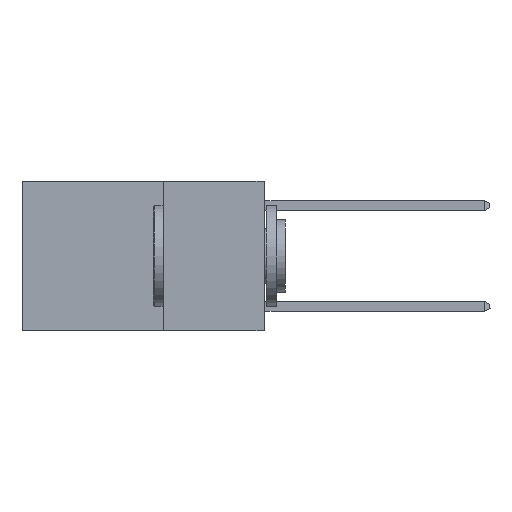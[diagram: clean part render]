
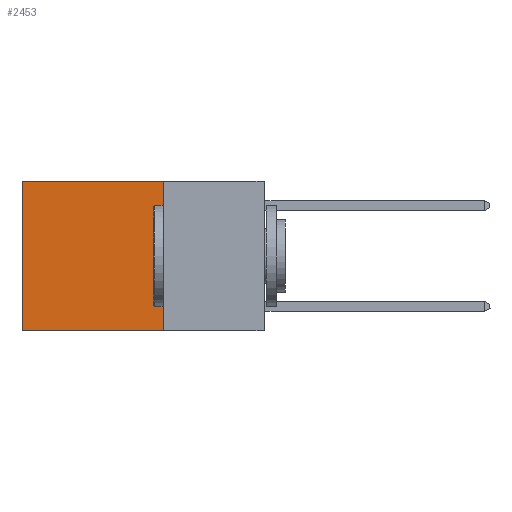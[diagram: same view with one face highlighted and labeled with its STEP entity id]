
A CAD part, left-side view. The second image highlights one B-rep face of the part: STEP entity #2453.
In plain terms, the highlighted planar face has unit normal (-1, 0, 0).
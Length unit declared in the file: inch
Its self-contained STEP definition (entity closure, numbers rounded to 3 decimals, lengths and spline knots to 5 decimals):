
#381 = DIRECTION ( 'NONE',  ( 1., 0., 0. ) ) ;
#887 = ORIENTED_EDGE ( 'NONE', *, *, #4737, .F. ) ;
#996 = LINE ( 'NONE', #11711, #10365 ) ;
#1130 = LINE ( 'NONE', #4098, #22455 ) ;
#1272 = CARTESIAN_POINT ( 'NONE',  ( 0.2625, 0.6, -0.37 ) ) ;
#1273 = CARTESIAN_POINT ( 'NONE',  ( 0.2625, 0.25, -0.37 ) ) ;
#1328 = CARTESIAN_POINT ( 'NONE',  ( 0.2625, 0.25, 0. ) ) ;
#2014 = FACE_OUTER_BOUND ( 'NONE', #2048, .T. ) ;
#2048 = EDGE_LOOP ( 'NONE', ( #14635, #13469, #887, #3648 ) ) ;
#2453 = ADVANCED_FACE ( 'NONE', ( #2014 ), #11058, .F. ) ;
#3527 = LINE ( 'NONE', #1328, #14250 ) ;
#3648 = ORIENTED_EDGE ( 'NONE', *, *, #15395, .T. ) ;
#4098 = CARTESIAN_POINT ( 'NONE',  ( 0.2625, 0.6, 0. ) ) ;
#4127 = VERTEX_POINT ( 'NONE', #8095 ) ;
#4737 = EDGE_CURVE ( 'NONE', #4127, #12629, #3527, .T. ) ;
#8095 = CARTESIAN_POINT ( 'NONE',  ( 0.2625, 0.25, 0. ) ) ;
#8576 = CARTESIAN_POINT ( 'NONE',  ( 0.2625, 0.6, 0. ) ) ;
#9661 = DIRECTION ( 'NONE',  ( 0., 1., 0. ) ) ;
#9745 = VERTEX_POINT ( 'NONE', #1272 ) ;
#9850 = DIRECTION ( 'NONE',  ( 0., 0., -1. ) ) ;
#10365 = VECTOR ( 'NONE', #9661, 39.37008 ) ;
#11058 = PLANE ( 'NONE',  #26579 ) ;
#11082 = DIRECTION ( 'NONE',  ( 0., 1., 0. ) ) ;
#11711 = CARTESIAN_POINT ( 'NONE',  ( 0.2625, 0.25, 0. ) ) ;
#12320 = EDGE_CURVE ( 'NONE', #12368, #9745, #1130, .T. ) ;
#12368 = VERTEX_POINT ( 'NONE', #8576 ) ;
#12530 = VECTOR ( 'NONE', #11082, 39.37008 ) ;
#12629 = VERTEX_POINT ( 'NONE', #1273 ) ;
#13469 = ORIENTED_EDGE ( 'NONE', *, *, #22594, .F. ) ;
#14250 = VECTOR ( 'NONE', #9850, 39.37008 ) ;
#14635 = ORIENTED_EDGE ( 'NONE', *, *, #12320, .T. ) ;
#14875 = DIRECTION ( 'NONE',  ( 0., 0., -1. ) ) ;
#15390 = DIRECTION ( 'NONE',  ( 0., 0., -1. ) ) ;
#15395 = EDGE_CURVE ( 'NONE', #4127, #12368, #996, .T. ) ;
#22455 = VECTOR ( 'NONE', #14875, 39.37008 ) ;
#22594 = EDGE_CURVE ( 'NONE', #12629, #9745, #25127, .T. ) ;
#23775 = CARTESIAN_POINT ( 'NONE',  ( 0.2625, 0.25, -0.37 ) ) ;
#25127 = LINE ( 'NONE', #23775, #12530 ) ;
#25900 = CARTESIAN_POINT ( 'NONE',  ( 0.2625, 0.25, 0. ) ) ;
#26579 = AXIS2_PLACEMENT_3D ( 'NONE', #25900, #381, #15390 ) ;
